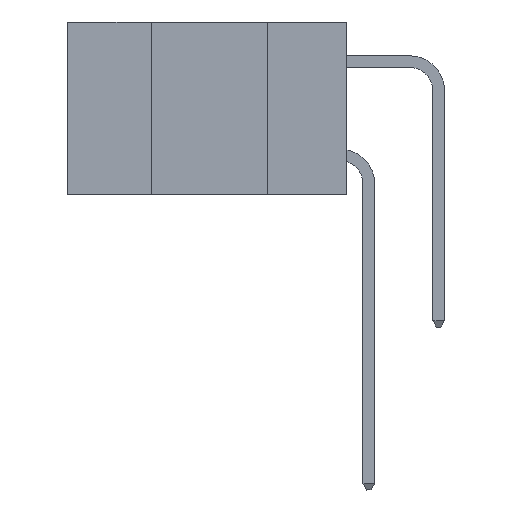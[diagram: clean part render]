
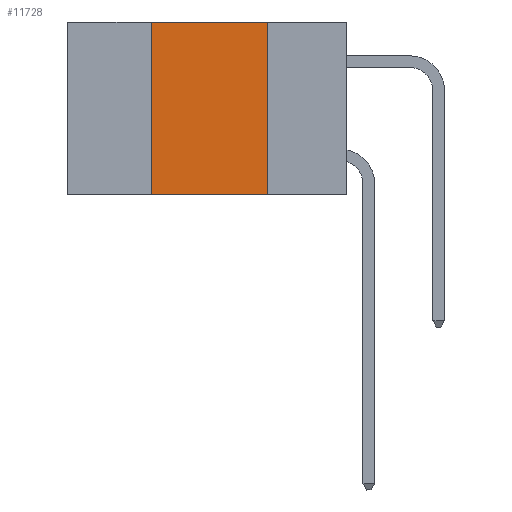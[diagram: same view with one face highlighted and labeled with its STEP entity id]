
A CAD part, left-side view. The second image highlights one B-rep face of the part: STEP entity #11728.
In plain terms, the highlighted planar face has unit normal (-1, 0, 0).
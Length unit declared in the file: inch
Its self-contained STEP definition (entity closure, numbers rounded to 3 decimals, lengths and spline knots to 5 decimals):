
#653 = VECTOR ( 'NONE', #13051, 39.37008 ) ;
#1085 = CARTESIAN_POINT ( 'NONE',  ( 0., 0.6, -0.37 ) ) ;
#1491 = EDGE_CURVE ( 'NONE', #8838, #1530, #4966, .T. ) ;
#1530 = VERTEX_POINT ( 'NONE', #18597 ) ;
#2062 = CARTESIAN_POINT ( 'NONE',  ( 0., 0.6, 0. ) ) ;
#2542 = ORIENTED_EDGE ( 'NONE', *, *, #12249, .F. ) ;
#2909 = LINE ( 'NONE', #1085, #21730 ) ;
#3391 = DIRECTION ( 'NONE',  ( 0., 0., 1. ) ) ;
#4399 = VERTEX_POINT ( 'NONE', #20869 ) ;
#4892 = DIRECTION ( 'NONE',  ( 0., 0., -1. ) ) ;
#4966 = LINE ( 'NONE', #2062, #653 ) ;
#5238 = EDGE_LOOP ( 'NONE', ( #2542, #6847, #7393, #8217 ) ) ;
#5750 = VECTOR ( 'NONE', #3391, 39.37008 ) ;
#6568 = DIRECTION ( 'NONE',  ( 0., -1., 0. ) ) ;
#6847 = ORIENTED_EDGE ( 'NONE', *, *, #1491, .F. ) ;
#6882 = CARTESIAN_POINT ( 'NONE',  ( 0., 0.42, 0. ) ) ;
#7025 = VERTEX_POINT ( 'NONE', #14717 ) ;
#7393 = ORIENTED_EDGE ( 'NONE', *, *, #22223, .F. ) ;
#7826 = CARTESIAN_POINT ( 'NONE',  ( 0., 0.6, 0. ) ) ;
#8217 = ORIENTED_EDGE ( 'NONE', *, *, #13444, .T. ) ;
#8561 = CARTESIAN_POINT ( 'NONE',  ( 0., 0.17, 0. ) ) ;
#8838 = VERTEX_POINT ( 'NONE', #6882 ) ;
#9681 = DIRECTION ( 'NONE',  ( 1., 0., 0. ) ) ;
#10630 = LINE ( 'NONE', #10695, #5750 ) ;
#10695 = CARTESIAN_POINT ( 'NONE',  ( 0., 0.42, 0. ) ) ;
#11728 = ADVANCED_FACE ( 'NONE', ( #18339 ), #18775, .F. ) ;
#12249 = EDGE_CURVE ( 'NONE', #1530, #7025, #21383, .T. ) ;
#13051 = DIRECTION ( 'NONE',  ( 0., -1., 0. ) ) ;
#13444 = EDGE_CURVE ( 'NONE', #4399, #7025, #2909, .T. ) ;
#14717 = CARTESIAN_POINT ( 'NONE',  ( 0., 0.17, -0.37 ) ) ;
#18339 = FACE_OUTER_BOUND ( 'NONE', #5238, .T. ) ;
#18597 = CARTESIAN_POINT ( 'NONE',  ( 0., 0.17, 0. ) ) ;
#18775 = PLANE ( 'NONE',  #21074 ) ;
#20869 = CARTESIAN_POINT ( 'NONE',  ( 0., 0.42, -0.37 ) ) ;
#21074 = AXIS2_PLACEMENT_3D ( 'NONE', #7826, #9681, #22379 ) ;
#21383 = LINE ( 'NONE', #8561, #21945 ) ;
#21730 = VECTOR ( 'NONE', #6568, 39.37008 ) ;
#21945 = VECTOR ( 'NONE', #4892, 39.37008 ) ;
#22223 = EDGE_CURVE ( 'NONE', #4399, #8838, #10630, .T. ) ;
#22379 = DIRECTION ( 'NONE',  ( 0., 0., -1. ) ) ;
